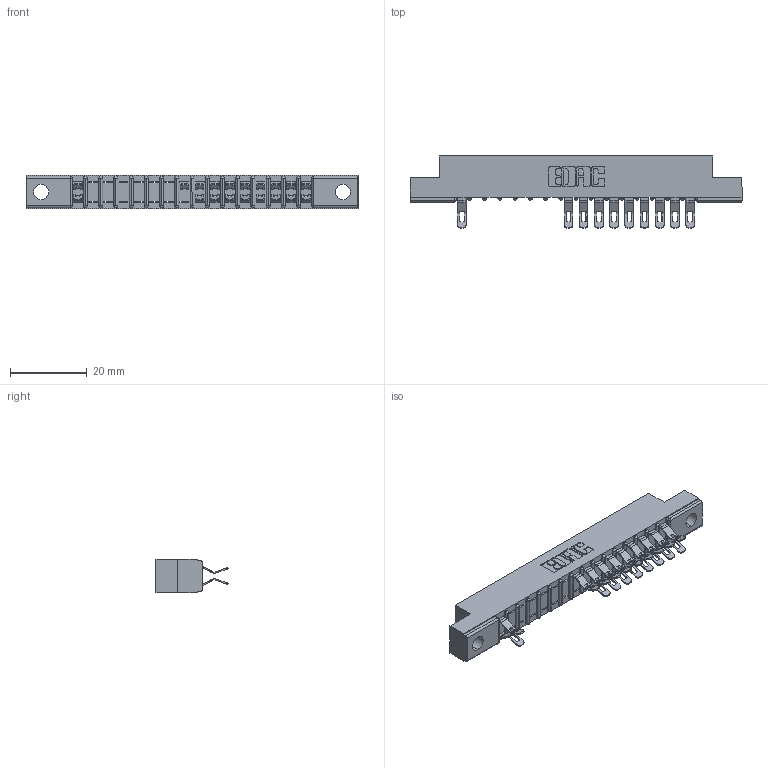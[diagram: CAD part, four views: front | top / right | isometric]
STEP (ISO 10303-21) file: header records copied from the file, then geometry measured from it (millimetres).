
FILE_DESCRIPTION (( 'STEP AP203' ), '1' );
FILE_NAME ('307-032-555-202.STEP', '2018-08-04T22:42:18', ( '' ), ( '' ), 'SwSTEP 2.0', 'SolidWorks 2016', '' );
FILE_SCHEMA (( 'CONFIG_CONTROL_DESIGN' ));
Length unit declared in the file: inch
Products named in the file (3): 307-290-001_555; 307-032-555-202; 307 Part_.128 Dia Mounting Holes
Assembly tree (20 placements, depth 2):
  307-032-555-202
    307 Part_.128 Dia Mounting Holes
    307-290-001_555  x19
Bounding box: 86.41 x 18.75 x 8.71 mm (x, y, z)
Volume: 5453.3 mm3; surface area: 8484.5 mm2
Topology: 20 solids, 20 shells, 1424 faces, 4178 edges, 2712 vertices
Faces by surface type: plane 794, cylinder 596, sphere 34
Entity records: 17557 total; most frequent: CARTESIAN_POINT 2939, ORIENTED_EDGE 2924, DIRECTION 2884, EDGE_CURVE 1462, LINE 1098, VECTOR 1098, VERTEX_POINT 948, AXIS2_PLACEMENT_3D 893
